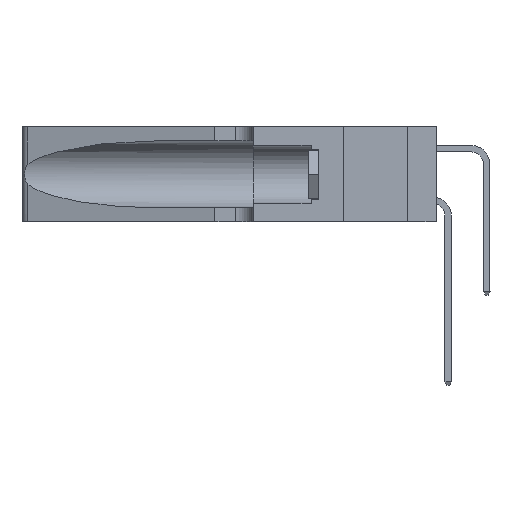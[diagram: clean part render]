
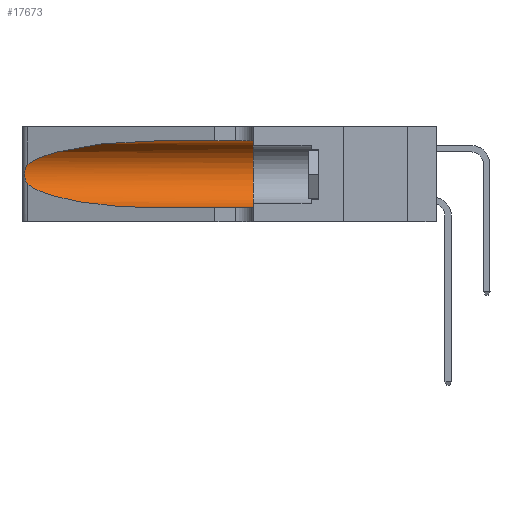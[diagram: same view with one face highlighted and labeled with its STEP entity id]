
A CAD part, left-side view. The second image highlights one B-rep face of the part: STEP entity #17673.
In plain terms, the highlighted cylindrical face has radius 3.308 mm (diameter 6.617 mm), a partial arc.
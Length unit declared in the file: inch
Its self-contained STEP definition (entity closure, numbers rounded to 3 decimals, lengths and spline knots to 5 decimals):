
#876 = CARTESIAN_POINT ( 'NONE',  ( 0.25856, 1.23593, 0.16098 ) ) ;
#1064 = CARTESIAN_POINT ( 'NONE',  ( 0.1305, 0.72297, 0.05475 ) ) ;
#2090 =( BOUNDED_CURVE ( )  B_SPLINE_CURVE ( 3, ( #16685, #24357, #20554, #8959 ),
 .UNSPECIFIED., .F., .F. ) 
 B_SPLINE_CURVE_WITH_KNOTS ( ( 4, 4 ),
 ( 1.5708, 2.84003 ),
 .UNSPECIFIED. ) 
 CURVE ( )  GEOMETRIC_REPRESENTATION_ITEM ( )  RATIONAL_B_SPLINE_CURVE ( ( 1., 0.87, 0.87, 1. ) ) 
 REPRESENTATION_ITEM ( '' )  );
#2259 = CARTESIAN_POINT ( 'NONE',  ( 0.1305, 0.72297, 0.31525 ) ) ;
#2363 = CARTESIAN_POINT ( 'NONE',  ( 0.1305, 1.61858, 0.185 ) ) ;
#2489 = CARTESIAN_POINT ( 'NONE',  ( 0.25487, 1.22718, 0.14631 ) ) ;
#2513 = CARTESIAN_POINT ( 'NONE',  ( 0.1305, 0.35, 0.31525 ) ) ;
#2557 = CARTESIAN_POINT ( 'NONE',  ( 0.1305, 0.35, 0.185 ) ) ;
#2887 = CARTESIAN_POINT ( 'NONE',  ( 0.25639, 1.23186, 0.15144 ) ) ;
#2923 = B_SPLINE_CURVE_WITH_KNOTS ( 'NONE', 3,
 ( #8655, #18414, #6780, #20327, #8736, #22266, #10688, #24220, #12628, #876, #14605, #2887, #16540, #4881 ),
 .UNSPECIFIED., .F., .F.,
 ( 4, 2, 2, 2, 2, 2, 4 ),
 ( 0., 0.00027, 0.00053, 0.00107, 0.0016, 0.00187, 0.00214 ),
 .UNSPECIFIED. ) ;
#3997 =( BOUNDED_CURVE ( )  B_SPLINE_CURVE ( 3, ( #22451, #24390, #12796, #1064 ),
 .UNSPECIFIED., .F., .F. ) 
 B_SPLINE_CURVE_WITH_KNOTS ( ( 4, 4 ),
 ( 3.44316, 4.71239 ),
 .UNSPECIFIED. ) 
 CURVE ( )  GEOMETRIC_REPRESENTATION_ITEM ( )  RATIONAL_B_SPLINE_CURVE ( ( 1., 0.87, 0.87, 1. ) ) 
 REPRESENTATION_ITEM ( '' )  );
#4546 = DIRECTION ( 'NONE',  ( 0., 0., 1. ) ) ;
#4827 = ORIENTED_EDGE ( 'NONE', *, *, #13276, .T. ) ;
#4881 = CARTESIAN_POINT ( 'NONE',  ( 0.25487, 1.22718, 0.14631 ) ) ;
#5209 = CIRCLE ( 'NONE', #20880, 0.13025 ) ;
#5380 = EDGE_CURVE ( 'NONE', #19805, #16933, #19771, .T. ) ;
#5862 = DIRECTION ( 'NONE',  ( 0., -1., 0. ) ) ;
#5979 = VERTEX_POINT ( 'NONE', #2259 ) ;
#6780 = CARTESIAN_POINT ( 'NONE',  ( 0.25639, 1.23184, 0.21858 ) ) ;
#6796 = VERTEX_POINT ( 'NONE', #2489 ) ;
#7152 = CYLINDRICAL_SURFACE ( 'NONE', #23258, 0.13025 ) ;
#8655 = CARTESIAN_POINT ( 'NONE',  ( 0.25487, 1.22718, 0.22369 ) ) ;
#8736 = CARTESIAN_POINT ( 'NONE',  ( 0.25854, 1.2359, 0.20912 ) ) ;
#8959 = CARTESIAN_POINT ( 'NONE',  ( 0.25487, 1.22718, 0.22369 ) ) ;
#9358 = CARTESIAN_POINT ( 'NONE',  ( 0.1305, 0.72297, 0.05475 ) ) ;
#9695 = CARTESIAN_POINT ( 'NONE',  ( 0.1305, 1.61858, 0.31525 ) ) ;
#10179 = DIRECTION ( 'NONE',  ( 0., -1., 0. ) ) ;
#10688 = CARTESIAN_POINT ( 'NONE',  ( 0.26075, 1.23896, 0.19203 ) ) ;
#10799 = EDGE_CURVE ( 'NONE', #5979, #18898, #10819, .T. ) ;
#10819 = LINE ( 'NONE', #9695, #15365 ) ;
#12044 = CARTESIAN_POINT ( 'NONE',  ( 0.1305, 1.61858, 0.05475 ) ) ;
#12370 = ORIENTED_EDGE ( 'NONE', *, *, #21897, .F. ) ;
#12628 = CARTESIAN_POINT ( 'NONE',  ( 0.26017, 1.23833, 0.17102 ) ) ;
#12796 = CARTESIAN_POINT ( 'NONE',  ( 0.18966, 0.96281, 0.05475 ) ) ;
#13276 = EDGE_CURVE ( 'NONE', #6796, #19805, #3997, .T. ) ;
#13328 = VERTEX_POINT ( 'NONE', #14932 ) ;
#13540 = ORIENTED_EDGE ( 'NONE', *, *, #16555, .T. ) ;
#14011 = VECTOR ( 'NONE', #21687, 39.37008 ) ;
#14134 = ORIENTED_EDGE ( 'NONE', *, *, #25160, .T. ) ;
#14422 = ORIENTED_EDGE ( 'NONE', *, *, #10799, .F. ) ;
#14605 = CARTESIAN_POINT ( 'NONE',  ( 0.25789, 1.23486, 0.15765 ) ) ;
#14932 = CARTESIAN_POINT ( 'NONE',  ( 0.25487, 1.22718, 0.22369 ) ) ;
#15365 = VECTOR ( 'NONE', #5862, 39.37008 ) ;
#16032 = DIRECTION ( 'NONE',  ( 0., 0., -1. ) ) ;
#16219 = DIRECTION ( 'NONE',  ( 0., 1., 0. ) ) ;
#16540 = CARTESIAN_POINT ( 'NONE',  ( 0.25555, 1.22993, 0.14849 ) ) ;
#16555 = EDGE_CURVE ( 'NONE', #5979, #13328, #2090, .T. ) ;
#16685 = CARTESIAN_POINT ( 'NONE',  ( 0.1305, 0.72297, 0.31525 ) ) ;
#16933 = VERTEX_POINT ( 'NONE', #23481 ) ;
#17673 = ADVANCED_FACE ( 'NONE', ( #18090 ), #7152, .F. ) ;
#18090 = FACE_OUTER_BOUND ( 'NONE', #23512, .T. ) ;
#18200 = ORIENTED_EDGE ( 'NONE', *, *, #5380, .T. ) ;
#18414 = CARTESIAN_POINT ( 'NONE',  ( 0.25555, 1.22994, 0.2215 ) ) ;
#18898 = VERTEX_POINT ( 'NONE', #2513 ) ;
#19771 = LINE ( 'NONE', #12044, #14011 ) ;
#19805 = VERTEX_POINT ( 'NONE', #9358 ) ;
#20327 = CARTESIAN_POINT ( 'NONE',  ( 0.25787, 1.23484, 0.2124 ) ) ;
#20554 = CARTESIAN_POINT ( 'NONE',  ( 0.2373, 1.15595, 0.28018 ) ) ;
#20880 = AXIS2_PLACEMENT_3D ( 'NONE', #2557, #16219, #4546 ) ;
#21687 = DIRECTION ( 'NONE',  ( 0., -1., 0. ) ) ;
#21897 = EDGE_CURVE ( 'NONE', #18898, #16933, #5209, .T. ) ;
#22266 = CARTESIAN_POINT ( 'NONE',  ( 0.26018, 1.23835, 0.19895 ) ) ;
#22451 = CARTESIAN_POINT ( 'NONE',  ( 0.25487, 1.22718, 0.14631 ) ) ;
#23258 = AXIS2_PLACEMENT_3D ( 'NONE', #2363, #10179, #16032 ) ;
#23481 = CARTESIAN_POINT ( 'NONE',  ( 0.1305, 0.35, 0.05475 ) ) ;
#23512 = EDGE_LOOP ( 'NONE', ( #13540, #14134, #4827, #18200, #12370, #14422 ) ) ;
#24220 = CARTESIAN_POINT ( 'NONE',  ( 0.26075, 1.23896, 0.178 ) ) ;
#24357 = CARTESIAN_POINT ( 'NONE',  ( 0.18966, 0.96281, 0.31525 ) ) ;
#24390 = CARTESIAN_POINT ( 'NONE',  ( 0.2373, 1.15595, 0.08982 ) ) ;
#25160 = EDGE_CURVE ( 'NONE', #13328, #6796, #2923, .T. ) ;
